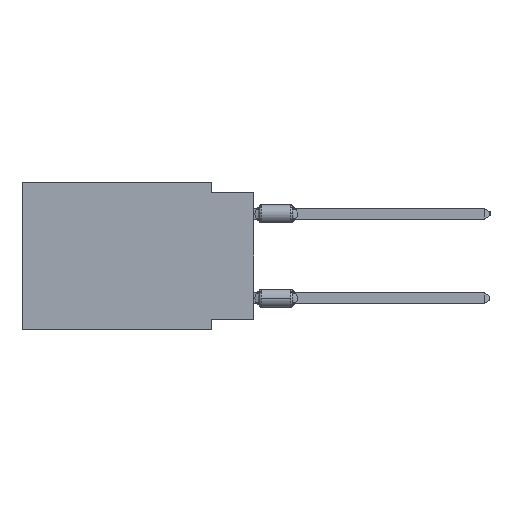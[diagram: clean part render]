
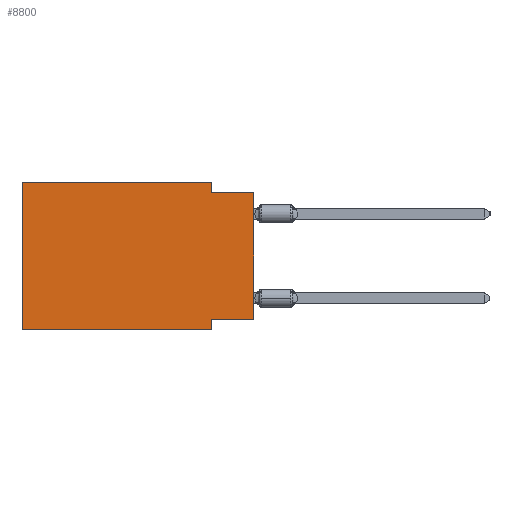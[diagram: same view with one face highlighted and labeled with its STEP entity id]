
A CAD part, left-side view. The second image highlights one B-rep face of the part: STEP entity #8800.
In plain terms, the highlighted planar face has unit normal (-1, 0, 0).
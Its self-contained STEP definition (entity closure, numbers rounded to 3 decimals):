
#2305 = VECTOR ( 'NONE', #5418, 1000. ) ;
#3616 = DIRECTION ( 'NONE',  ( 0., -1., 0. ) ) ;
#3628 = VERTEX_POINT ( 'NONE', #9107 ) ;
#4284 = DIRECTION ( 'NONE',  ( 0., 0., -1. ) ) ;
#4679 = EDGE_CURVE ( 'NONE', #16920, #32337, #11034, .T. ) ;
#5418 = DIRECTION ( 'NONE',  ( 0., -1., 0. ) ) ;
#7684 = VERTEX_POINT ( 'NONE', #8186 ) ;
#7705 = CARTESIAN_POINT ( 'NONE',  ( 0., 0., -8.255 ) ) ;
#7706 = CARTESIAN_POINT ( 'NONE',  ( 0., 13.97, 0. ) ) ;
#7852 = CARTESIAN_POINT ( 'NONE',  ( 0., 2.54, -8.89 ) ) ;
#7887 = DIRECTION ( 'NONE',  ( 0., 1., 0. ) ) ;
#8040 = VECTOR ( 'NONE', #38339, 1000. ) ;
#8186 = CARTESIAN_POINT ( 'NONE',  ( 0., 2.54, 0. ) ) ;
#8800 = ADVANCED_FACE ( 'NONE', ( #23327 ), #35332, .F. ) ;
#8844 = DIRECTION ( 'NONE',  ( 0., 0., -1. ) ) ;
#9107 = CARTESIAN_POINT ( 'NONE',  ( 0., 0., -0.635 ) ) ;
#9411 = CARTESIAN_POINT ( 'NONE',  ( 0., 2.54, -0.635 ) ) ;
#9765 = ORIENTED_EDGE ( 'NONE', *, *, #25875, .F. ) ;
#10346 = EDGE_CURVE ( 'NONE', #29583, #35235, #22625, .T. ) ;
#10588 = ORIENTED_EDGE ( 'NONE', *, *, #10346, .F. ) ;
#11034 = LINE ( 'NONE', #7706, #23568 ) ;
#11133 = DIRECTION ( 'NONE',  ( 0., -1., 0. ) ) ;
#11794 = LINE ( 'NONE', #14740, #8040 ) ;
#12333 = EDGE_CURVE ( 'NONE', #22939, #3628, #23294, .T. ) ;
#12383 = CARTESIAN_POINT ( 'NONE',  ( 0., 2.54, 0. ) ) ;
#12653 = CARTESIAN_POINT ( 'NONE',  ( 0., 13.97, -8.89 ) ) ;
#12748 = ORIENTED_EDGE ( 'NONE', *, *, #4679, .F. ) ;
#14445 = VECTOR ( 'NONE', #8844, 1000. ) ;
#14670 = CARTESIAN_POINT ( 'NONE',  ( 0., 0., -0.635 ) ) ;
#14740 = CARTESIAN_POINT ( 'NONE',  ( 0., 0., 0. ) ) ;
#15519 = VERTEX_POINT ( 'NONE', #7852 ) ;
#15601 = EDGE_LOOP ( 'NONE', ( #19597, #20781, #35283, #17821, #12748, #31903, #9765, #10588 ) ) ;
#15718 = VECTOR ( 'NONE', #11133, 1000. ) ;
#16612 = CARTESIAN_POINT ( 'NONE',  ( 0., 13.97, -8.89 ) ) ;
#16920 = VERTEX_POINT ( 'NONE', #16612 ) ;
#17821 = ORIENTED_EDGE ( 'NONE', *, *, #26511, .F. ) ;
#17883 = LINE ( 'NONE', #12383, #31974 ) ;
#19597 = ORIENTED_EDGE ( 'NONE', *, *, #24030, .T. ) ;
#20201 = DIRECTION ( 'NONE',  ( 0., 0., -1. ) ) ;
#20360 = LINE ( 'NONE', #38252, #2305 ) ;
#20781 = ORIENTED_EDGE ( 'NONE', *, *, #12333, .F. ) ;
#21733 = VECTOR ( 'NONE', #3616, 1000. ) ;
#22625 = LINE ( 'NONE', #7705, #26467 ) ;
#22939 = VERTEX_POINT ( 'NONE', #9411 ) ;
#23294 = LINE ( 'NONE', #14670, #15718 ) ;
#23327 = FACE_OUTER_BOUND ( 'NONE', #15601, .T. ) ;
#23568 = VECTOR ( 'NONE', #37391, 1000. ) ;
#24030 = EDGE_CURVE ( 'NONE', #29583, #3628, #11794, .T. ) ;
#24263 = CARTESIAN_POINT ( 'NONE',  ( 0., 13.97, 0. ) ) ;
#25875 = EDGE_CURVE ( 'NONE', #35235, #15519, #33193, .T. ) ;
#26448 = CARTESIAN_POINT ( 'NONE',  ( 0., 0., -8.255 ) ) ;
#26467 = VECTOR ( 'NONE', #7887, 1000. ) ;
#26511 = EDGE_CURVE ( 'NONE', #32337, #7684, #20360, .T. ) ;
#28851 = DIRECTION ( 'NONE',  ( 1., 0., 0. ) ) ;
#29583 = VERTEX_POINT ( 'NONE', #26448 ) ;
#30441 = CARTESIAN_POINT ( 'NONE',  ( 0., 2.54, -8.89 ) ) ;
#30732 = CARTESIAN_POINT ( 'NONE',  ( 0., 2.54, -8.255 ) ) ;
#31903 = ORIENTED_EDGE ( 'NONE', *, *, #36463, .T. ) ;
#31974 = VECTOR ( 'NONE', #4284, 1000. ) ;
#32337 = VERTEX_POINT ( 'NONE', #24263 ) ;
#33193 = LINE ( 'NONE', #30441, #14445 ) ;
#33333 = EDGE_CURVE ( 'NONE', #7684, #22939, #17883, .T. ) ;
#35235 = VERTEX_POINT ( 'NONE', #30732 ) ;
#35283 = ORIENTED_EDGE ( 'NONE', *, *, #33333, .F. ) ;
#35332 = PLANE ( 'NONE',  #37157 ) ;
#36463 = EDGE_CURVE ( 'NONE', #16920, #15519, #36840, .T. ) ;
#36840 = LINE ( 'NONE', #12653, #21733 ) ;
#37157 = AXIS2_PLACEMENT_3D ( 'NONE', #37511, #28851, #20201 ) ;
#37391 = DIRECTION ( 'NONE',  ( 0., 0., 1. ) ) ;
#37511 = CARTESIAN_POINT ( 'NONE',  ( 0., 13.97, 0. ) ) ;
#38252 = CARTESIAN_POINT ( 'NONE',  ( 0., 13.97, 0. ) ) ;
#38339 = DIRECTION ( 'NONE',  ( 0., 0., 1. ) ) ;
